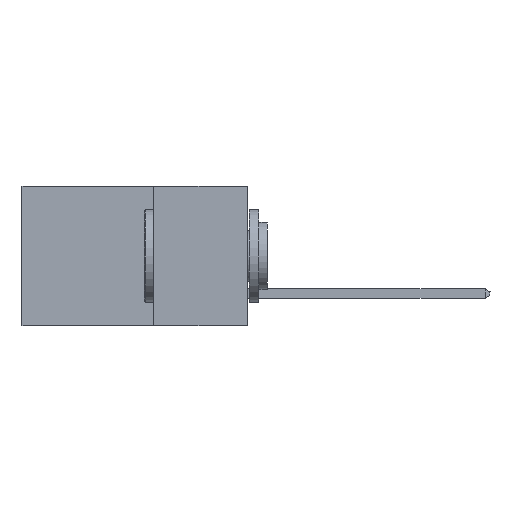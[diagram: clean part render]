
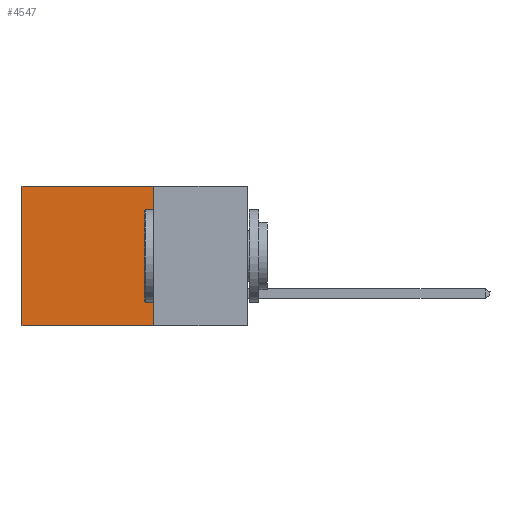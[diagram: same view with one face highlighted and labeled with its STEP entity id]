
A CAD part, left-side view. The second image highlights one B-rep face of the part: STEP entity #4547.
In plain terms, the highlighted planar face has unit normal (-1, 0, 0).
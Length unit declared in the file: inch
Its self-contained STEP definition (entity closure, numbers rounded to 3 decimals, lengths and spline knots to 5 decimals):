
#70 = EDGE_LOOP ( 'NONE', ( #157, #7281, #17901, #4845 ) ) ;
#157 = ORIENTED_EDGE ( 'NONE', *, *, #11050, .T. ) ;
#1379 = EDGE_CURVE ( 'NONE', #12575, #5127, #8682, .T. ) ;
#1485 = CARTESIAN_POINT ( 'NONE',  ( 0.2615, 0.6, -0.37 ) ) ;
#2323 = LINE ( 'NONE', #13881, #17055 ) ;
#3851 = DIRECTION ( 'NONE',  ( 0., 0., -1. ) ) ;
#4101 = CARTESIAN_POINT ( 'NONE',  ( 0.2615, 0.25, -0.37 ) ) ;
#4410 = DIRECTION ( 'NONE',  ( 0., 0., -1. ) ) ;
#4547 = ADVANCED_FACE ( 'NONE', ( #20973 ), #6046, .F. ) ;
#4731 = CARTESIAN_POINT ( 'NONE',  ( 0.2615, 0.25, -0.37 ) ) ;
#4812 = DIRECTION ( 'NONE',  ( 0., 1., 0. ) ) ;
#4845 = ORIENTED_EDGE ( 'NONE', *, *, #7345, .T. ) ;
#5127 = VERTEX_POINT ( 'NONE', #1485 ) ;
#6046 = PLANE ( 'NONE',  #13381 ) ;
#6371 = VECTOR ( 'NONE', #15345, 39.37008 ) ;
#7205 = EDGE_CURVE ( 'NONE', #11021, #12575, #2323, .T. ) ;
#7281 = ORIENTED_EDGE ( 'NONE', *, *, #1379, .F. ) ;
#7345 = EDGE_CURVE ( 'NONE', #11021, #13438, #20957, .T. ) ;
#7974 = CARTESIAN_POINT ( 'NONE',  ( 0.2615, 0.25, 0. ) ) ;
#8682 = LINE ( 'NONE', #4101, #6371 ) ;
#9072 = CARTESIAN_POINT ( 'NONE',  ( 0.2615, 0.25, -0.37 ) ) ;
#11021 = VERTEX_POINT ( 'NONE', #14852 ) ;
#11050 = EDGE_CURVE ( 'NONE', #13438, #5127, #16593, .T. ) ;
#11359 = DIRECTION ( 'NONE',  ( 0., 0., -1. ) ) ;
#11389 = CARTESIAN_POINT ( 'NONE',  ( 0.2615, 0.6, 0. ) ) ;
#12575 = VERTEX_POINT ( 'NONE', #9072 ) ;
#12600 = VECTOR ( 'NONE', #11359, 39.37008 ) ;
#12698 = DIRECTION ( 'NONE',  ( 1., 0., 0. ) ) ;
#13209 = CARTESIAN_POINT ( 'NONE',  ( 0.2615, 0.6, -0.37 ) ) ;
#13381 = AXIS2_PLACEMENT_3D ( 'NONE', #4731, #12698, #4410 ) ;
#13438 = VERTEX_POINT ( 'NONE', #11389 ) ;
#13881 = CARTESIAN_POINT ( 'NONE',  ( 0.2615, 0.25, -0.37 ) ) ;
#14852 = CARTESIAN_POINT ( 'NONE',  ( 0.2615, 0.25, 0. ) ) ;
#15345 = DIRECTION ( 'NONE',  ( 0., 1., 0. ) ) ;
#16593 = LINE ( 'NONE', #13209, #12600 ) ;
#17055 = VECTOR ( 'NONE', #3851, 39.37008 ) ;
#17901 = ORIENTED_EDGE ( 'NONE', *, *, #7205, .F. ) ;
#19844 = VECTOR ( 'NONE', #4812, 39.37008 ) ;
#20957 = LINE ( 'NONE', #7974, #19844 ) ;
#20973 = FACE_OUTER_BOUND ( 'NONE', #70, .T. ) ;
